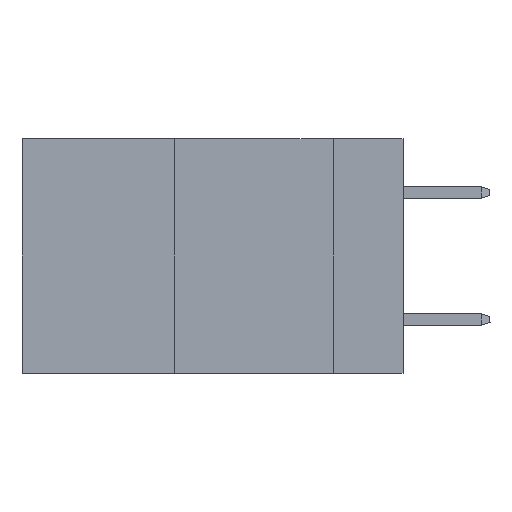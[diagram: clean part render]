
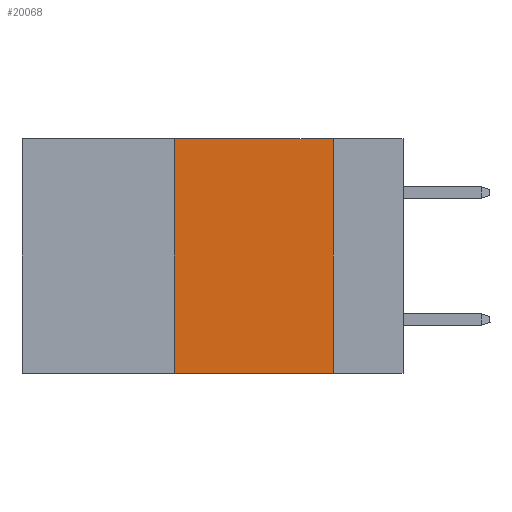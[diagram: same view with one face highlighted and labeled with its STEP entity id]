
A CAD part, left-side view. The second image highlights one B-rep face of the part: STEP entity #20068.
In plain terms, the highlighted planar face has unit normal (-1, 0, 0).
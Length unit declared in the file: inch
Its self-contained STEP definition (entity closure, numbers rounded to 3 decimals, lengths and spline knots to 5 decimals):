
#391 = LINE ( 'NONE', #14645, #1392 ) ;
#661 = VECTOR ( 'NONE', #14726, 39.37008 ) ;
#1392 = VECTOR ( 'NONE', #10630, 39.37008 ) ;
#2212 = VERTEX_POINT ( 'NONE', #25907 ) ;
#2280 = ORIENTED_EDGE ( 'NONE', *, *, #7698, .F. ) ;
#3127 = PLANE ( 'NONE',  #9508 ) ;
#4110 = ORIENTED_EDGE ( 'NONE', *, *, #19506, .F. ) ;
#7021 = FACE_OUTER_BOUND ( 'NONE', #20013, .T. ) ;
#7698 = EDGE_CURVE ( 'NONE', #2212, #16290, #391, .T. ) ;
#9434 = DIRECTION ( 'NONE',  ( 0., 0., -1. ) ) ;
#9508 = AXIS2_PLACEMENT_3D ( 'NONE', #21750, #17763, #9434 ) ;
#9863 = VECTOR ( 'NONE', #20615, 39.37008 ) ;
#10016 = EDGE_CURVE ( 'NONE', #19038, #24759, #12312, .T. ) ;
#10630 = DIRECTION ( 'NONE',  ( 0., 0., -1. ) ) ;
#12312 = LINE ( 'NONE', #24937, #661 ) ;
#13592 = LINE ( 'NONE', #17643, #20238 ) ;
#14645 = CARTESIAN_POINT ( 'NONE',  ( 0., 0.11, 0. ) ) ;
#14726 = DIRECTION ( 'NONE',  ( 0., 0., 1. ) ) ;
#16290 = VERTEX_POINT ( 'NONE', #19482 ) ;
#16802 = EDGE_CURVE ( 'NONE', #19038, #16290, #18338, .T. ) ;
#17643 = CARTESIAN_POINT ( 'NONE',  ( 0., 0.6, 0. ) ) ;
#17763 = DIRECTION ( 'NONE',  ( 1., 0., 0. ) ) ;
#18338 = LINE ( 'NONE', #24125, #9863 ) ;
#19038 = VERTEX_POINT ( 'NONE', #20837 ) ;
#19482 = CARTESIAN_POINT ( 'NONE',  ( 0., 0.11, -0.37 ) ) ;
#19506 = EDGE_CURVE ( 'NONE', #24759, #2212, #13592, .T. ) ;
#19747 = DIRECTION ( 'NONE',  ( 0., -1., 0. ) ) ;
#20013 = EDGE_LOOP ( 'NONE', ( #2280, #4110, #22397, #24733 ) ) ;
#20068 = ADVANCED_FACE ( 'NONE', ( #7021 ), #3127, .F. ) ;
#20238 = VECTOR ( 'NONE', #19747, 39.37008 ) ;
#20615 = DIRECTION ( 'NONE',  ( 0., -1., 0. ) ) ;
#20837 = CARTESIAN_POINT ( 'NONE',  ( 0., 0.36, -0.37 ) ) ;
#21750 = CARTESIAN_POINT ( 'NONE',  ( 0., 0.6, 0. ) ) ;
#22397 = ORIENTED_EDGE ( 'NONE', *, *, #10016, .F. ) ;
#23168 = CARTESIAN_POINT ( 'NONE',  ( 0., 0.36, 0. ) ) ;
#24125 = CARTESIAN_POINT ( 'NONE',  ( 0., 0.6, -0.37 ) ) ;
#24733 = ORIENTED_EDGE ( 'NONE', *, *, #16802, .T. ) ;
#24759 = VERTEX_POINT ( 'NONE', #23168 ) ;
#24937 = CARTESIAN_POINT ( 'NONE',  ( 0., 0.36, 0. ) ) ;
#25907 = CARTESIAN_POINT ( 'NONE',  ( 0., 0.11, 0. ) ) ;
